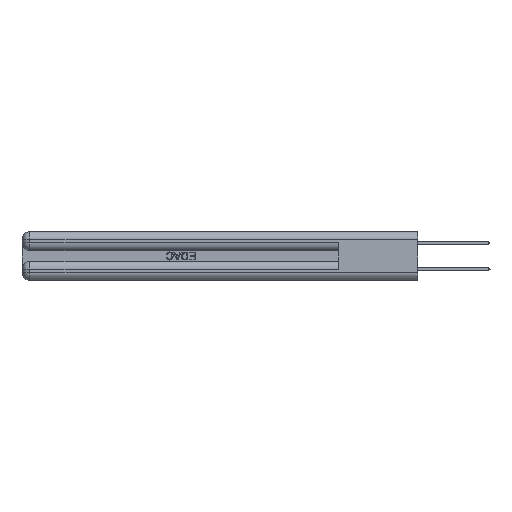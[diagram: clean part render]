
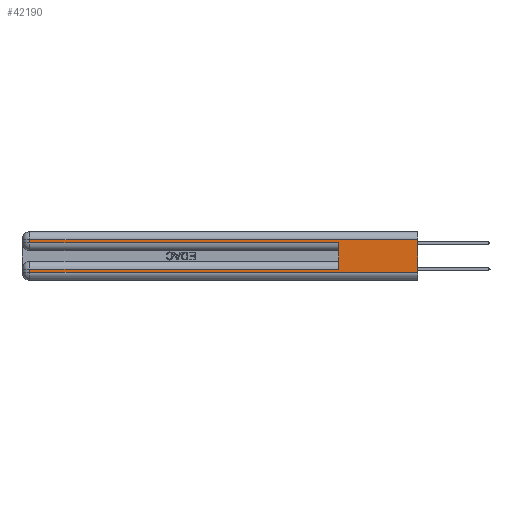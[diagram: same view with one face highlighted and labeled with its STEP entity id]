
A CAD part, left-side view. The second image highlights one B-rep face of the part: STEP entity #42190.
In plain terms, the highlighted planar face has unit normal (-1, 0, 0).
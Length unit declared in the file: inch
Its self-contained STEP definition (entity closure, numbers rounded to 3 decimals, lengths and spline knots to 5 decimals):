
#759 = LINE ( 'NONE', #31734, #11478 ) ;
#1233 = VECTOR ( 'NONE', #15961, 39.37008 ) ;
#2702 = LINE ( 'NONE', #6195, #12136 ) ;
#3151 = VERTEX_POINT ( 'NONE', #27418 ) ;
#3868 = LINE ( 'NONE', #42193, #24024 ) ;
#5515 = EDGE_CURVE ( 'NONE', #46051, #25914, #2702, .T. ) ;
#5757 = EDGE_CURVE ( 'NONE', #22479, #46051, #759, .T. ) ;
#6195 = CARTESIAN_POINT ( 'NONE',  ( 0., 2.94, 0.37 ) ) ;
#7202 = CARTESIAN_POINT ( 'NONE',  ( 0., 0.6, 0.285 ) ) ;
#7379 = EDGE_CURVE ( 'NONE', #11494, #3151, #42589, .T. ) ;
#7642 = CARTESIAN_POINT ( 'NONE',  ( 0., 0., 0.37 ) ) ;
#7706 = DIRECTION ( 'NONE',  ( 0., 1., 0. ) ) ;
#7716 = EDGE_CURVE ( 'NONE', #18753, #39095, #48776, .T. ) ;
#7815 = DIRECTION ( 'NONE',  ( 1., 0., 0. ) ) ;
#7953 = EDGE_CURVE ( 'NONE', #25914, #39095, #49381, .T. ) ;
#8164 = CARTESIAN_POINT ( 'NONE',  ( 0., 2.94, 0.285 ) ) ;
#8852 = ORIENTED_EDGE ( 'NONE', *, *, #7379, .T. ) ;
#10237 = DIRECTION ( 'NONE',  ( 0., 0., -1. ) ) ;
#11478 = VECTOR ( 'NONE', #7706, 39.37008 ) ;
#11494 = VERTEX_POINT ( 'NONE', #23696 ) ;
#11957 = ORIENTED_EDGE ( 'NONE', *, *, #51805, .F. ) ;
#12136 = VECTOR ( 'NONE', #10237, 39.37008 ) ;
#12588 = ORIENTED_EDGE ( 'NONE', *, *, #7716, .F. ) ;
#12606 = ORIENTED_EDGE ( 'NONE', *, *, #5757, .T. ) ;
#14672 = FACE_OUTER_BOUND ( 'NONE', #47728, .T. ) ;
#15066 = LINE ( 'NONE', #43925, #36300 ) ;
#15365 = CARTESIAN_POINT ( 'NONE',  ( 0., 0., 0.285 ) ) ;
#15961 = DIRECTION ( 'NONE',  ( 0., 0., -1. ) ) ;
#16018 = DIRECTION ( 'NONE',  ( 0., 0., -1. ) ) ;
#16172 = DIRECTION ( 'NONE',  ( 0., 1., 0. ) ) ;
#17576 = VECTOR ( 'NONE', #43281, 39.37008 ) ;
#18753 = VERTEX_POINT ( 'NONE', #35737 ) ;
#19561 = ORIENTED_EDGE ( 'NONE', *, *, #5515, .T. ) ;
#20536 = VERTEX_POINT ( 'NONE', #43347 ) ;
#21292 = ORIENTED_EDGE ( 'NONE', *, *, #35445, .T. ) ;
#22479 = VERTEX_POINT ( 'NONE', #35871 ) ;
#23696 = CARTESIAN_POINT ( 'NONE',  ( 0., 2.94, 0.085 ) ) ;
#24024 = VECTOR ( 'NONE', #34325, 39.37008 ) ;
#25914 = VERTEX_POINT ( 'NONE', #8164 ) ;
#27418 = CARTESIAN_POINT ( 'NONE',  ( 0., 2.94, 0.06 ) ) ;
#27473 = AXIS2_PLACEMENT_3D ( 'NONE', #7642, #7815, #35828 ) ;
#29960 = DIRECTION ( 'NONE',  ( 0., 0., 1. ) ) ;
#31615 = LINE ( 'NONE', #40073, #42234 ) ;
#31734 = CARTESIAN_POINT ( 'NONE',  ( 0., 0., 0.31 ) ) ;
#31832 = PLANE ( 'NONE',  #27473 ) ;
#34324 = ORIENTED_EDGE ( 'NONE', *, *, #7953, .T. ) ;
#34325 = DIRECTION ( 'NONE',  ( 0., -1., 0. ) ) ;
#35445 = EDGE_CURVE ( 'NONE', #18753, #11494, #31615, .T. ) ;
#35737 = CARTESIAN_POINT ( 'NONE',  ( 0., 0.6, 0.085 ) ) ;
#35828 = DIRECTION ( 'NONE',  ( 0., 0., -1. ) ) ;
#35871 = CARTESIAN_POINT ( 'NONE',  ( 0., 0., 0.31 ) ) ;
#36300 = VECTOR ( 'NONE', #16018, 39.37008 ) ;
#36330 = CARTESIAN_POINT ( 'NONE',  ( 0., 2.94, 0.31 ) ) ;
#36915 = VECTOR ( 'NONE', #29960, 39.37008 ) ;
#39095 = VERTEX_POINT ( 'NONE', #7202 ) ;
#40073 = CARTESIAN_POINT ( 'NONE',  ( 0., 0., 0.085 ) ) ;
#42190 = ADVANCED_FACE ( 'NONE', ( #14672 ), #31832, .F. ) ;
#42193 = CARTESIAN_POINT ( 'NONE',  ( 0., 0., 0.06 ) ) ;
#42234 = VECTOR ( 'NONE', #16172, 39.37008 ) ;
#42589 = LINE ( 'NONE', #43860, #1233 ) ;
#43281 = DIRECTION ( 'NONE',  ( 0., -1., 0. ) ) ;
#43347 = CARTESIAN_POINT ( 'NONE',  ( 0., 0., 0.06 ) ) ;
#43860 = CARTESIAN_POINT ( 'NONE',  ( 0., 2.94, 0.37 ) ) ;
#43925 = CARTESIAN_POINT ( 'NONE',  ( 0., 0., 0.37 ) ) ;
#46051 = VERTEX_POINT ( 'NONE', #36330 ) ;
#47152 = ORIENTED_EDGE ( 'NONE', *, *, #50215, .T. ) ;
#47728 = EDGE_LOOP ( 'NONE', ( #11957, #12606, #19561, #34324, #12588, #21292, #8852, #47152 ) ) ;
#48776 = LINE ( 'NONE', #49772, #36915 ) ;
#49381 = LINE ( 'NONE', #15365, #17576 ) ;
#49772 = CARTESIAN_POINT ( 'NONE',  ( 0., 0.6, 0.145 ) ) ;
#50215 = EDGE_CURVE ( 'NONE', #3151, #20536, #3868, .T. ) ;
#51805 = EDGE_CURVE ( 'NONE', #22479, #20536, #15066, .T. ) ;
